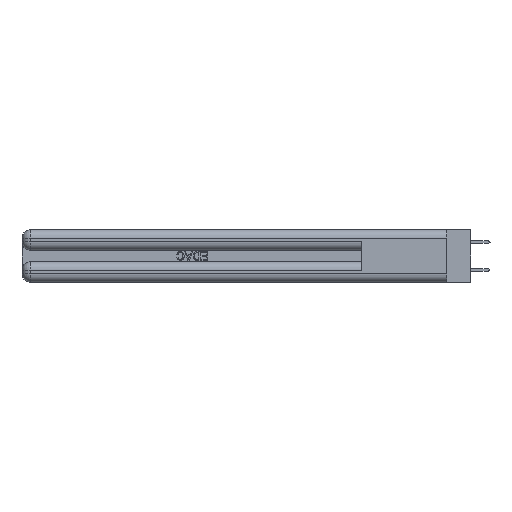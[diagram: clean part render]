
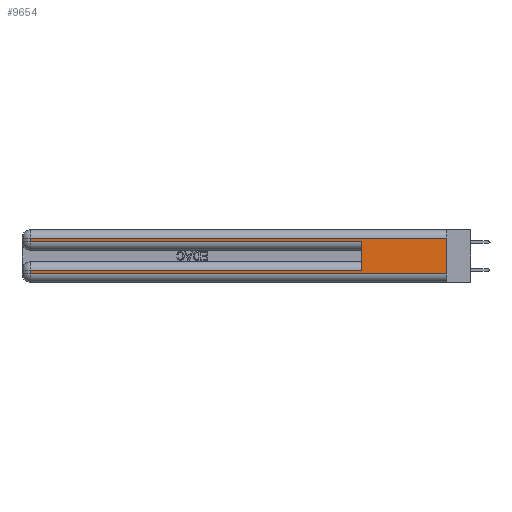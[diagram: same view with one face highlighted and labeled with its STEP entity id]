
A CAD part, left-side view. The second image highlights one B-rep face of the part: STEP entity #9654.
In plain terms, the highlighted planar face has unit normal (-1, 0, 0).
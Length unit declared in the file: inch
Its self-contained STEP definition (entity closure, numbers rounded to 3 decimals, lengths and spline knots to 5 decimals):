
#484 = CARTESIAN_POINT ( 'NONE',  ( 0., 0.6, 0.145 ) ) ;
#1124 = CARTESIAN_POINT ( 'NONE',  ( 0., 2.94, 0.37 ) ) ;
#2005 = VERTEX_POINT ( 'NONE', #11584 ) ;
#2171 = LINE ( 'NONE', #6104, #13094 ) ;
#2216 = DIRECTION ( 'NONE',  ( 0., 0., -1. ) ) ;
#2719 = VECTOR ( 'NONE', #2216, 39.37008 ) ;
#3915 = ORIENTED_EDGE ( 'NONE', *, *, #27995, .T. ) ;
#4435 = EDGE_CURVE ( 'NONE', #2005, #12462, #10075, .T. ) ;
#5364 = DIRECTION ( 'NONE',  ( 1., 0., 0. ) ) ;
#6104 = CARTESIAN_POINT ( 'NONE',  ( 0., 0., 0.06 ) ) ;
#6538 = ORIENTED_EDGE ( 'NONE', *, *, #22815, .T. ) ;
#6700 = EDGE_CURVE ( 'NONE', #31716, #38240, #8829, .T. ) ;
#7305 = DIRECTION ( 'NONE',  ( 0., -1., 0. ) ) ;
#7788 = CARTESIAN_POINT ( 'NONE',  ( 0., 2.94, 0.37 ) ) ;
#8379 = VECTOR ( 'NONE', #30984, 39.37008 ) ;
#8384 = DIRECTION ( 'NONE',  ( 0., -1., 0. ) ) ;
#8829 = LINE ( 'NONE', #21526, #8379 ) ;
#9579 = ORIENTED_EDGE ( 'NONE', *, *, #6700, .T. ) ;
#9654 = ADVANCED_FACE ( 'NONE', ( #11792 ), #26966, .F. ) ;
#9795 = VECTOR ( 'NONE', #15200, 39.37008 ) ;
#9812 = LINE ( 'NONE', #32576, #33834 ) ;
#10075 = LINE ( 'NONE', #484, #14233 ) ;
#11584 = CARTESIAN_POINT ( 'NONE',  ( 0., 0.6, 0.085 ) ) ;
#11792 = FACE_OUTER_BOUND ( 'NONE', #14439, .T. ) ;
#12462 = VERTEX_POINT ( 'NONE', #17905 ) ;
#12486 = EDGE_CURVE ( 'NONE', #35763, #12462, #9812, .T. ) ;
#13094 = VECTOR ( 'NONE', #8384, 39.37008 ) ;
#13148 = AXIS2_PLACEMENT_3D ( 'NONE', #36479, #5364, #20777 ) ;
#14137 = ORIENTED_EDGE ( 'NONE', *, *, #4435, .F. ) ;
#14233 = VECTOR ( 'NONE', #20050, 39.37008 ) ;
#14439 = EDGE_LOOP ( 'NONE', ( #24627, #9579, #3915, #22885, #14137, #6538, #19236, #23419 ) ) ;
#15200 = DIRECTION ( 'NONE',  ( 0., 1., 0. ) ) ;
#15287 = LINE ( 'NONE', #21546, #2719 ) ;
#16349 = VERTEX_POINT ( 'NONE', #16512 ) ;
#16512 = CARTESIAN_POINT ( 'NONE',  ( 0., 2.94, 0.085 ) ) ;
#17905 = CARTESIAN_POINT ( 'NONE',  ( 0., 0.6, 0.285 ) ) ;
#18351 = LINE ( 'NONE', #28795, #9795 ) ;
#19073 = CARTESIAN_POINT ( 'NONE',  ( 0., 2.94, 0.31 ) ) ;
#19236 = ORIENTED_EDGE ( 'NONE', *, *, #37126, .T. ) ;
#19526 = CARTESIAN_POINT ( 'NONE',  ( 0., 2.94, 0.285 ) ) ;
#20050 = DIRECTION ( 'NONE',  ( 0., 0., 1. ) ) ;
#20777 = DIRECTION ( 'NONE',  ( 0., 0., -1. ) ) ;
#21146 = CARTESIAN_POINT ( 'NONE',  ( 0., 2.94, 0.06 ) ) ;
#21526 = CARTESIAN_POINT ( 'NONE',  ( 0., 0., 0.31 ) ) ;
#21546 = CARTESIAN_POINT ( 'NONE',  ( 0., 0., 0.37 ) ) ;
#21895 = VECTOR ( 'NONE', #39509, 39.37008 ) ;
#22815 = EDGE_CURVE ( 'NONE', #2005, #16349, #18351, .T. ) ;
#22885 = ORIENTED_EDGE ( 'NONE', *, *, #12486, .T. ) ;
#23309 = EDGE_CURVE ( 'NONE', #33878, #38286, #2171, .T. ) ;
#23384 = LINE ( 'NONE', #7788, #21895 ) ;
#23419 = ORIENTED_EDGE ( 'NONE', *, *, #23309, .T. ) ;
#24627 = ORIENTED_EDGE ( 'NONE', *, *, #29387, .F. ) ;
#26156 = VECTOR ( 'NONE', #29727, 39.37008 ) ;
#26966 = PLANE ( 'NONE',  #13148 ) ;
#27995 = EDGE_CURVE ( 'NONE', #38240, #35763, #23384, .T. ) ;
#28795 = CARTESIAN_POINT ( 'NONE',  ( 0., 0., 0.085 ) ) ;
#29387 = EDGE_CURVE ( 'NONE', #31716, #38286, #15287, .T. ) ;
#29528 = LINE ( 'NONE', #1124, #26156 ) ;
#29727 = DIRECTION ( 'NONE',  ( 0., 0., -1. ) ) ;
#30984 = DIRECTION ( 'NONE',  ( 0., 1., 0. ) ) ;
#31716 = VERTEX_POINT ( 'NONE', #38873 ) ;
#32576 = CARTESIAN_POINT ( 'NONE',  ( 0., 0., 0.285 ) ) ;
#33834 = VECTOR ( 'NONE', #7305, 39.37008 ) ;
#33878 = VERTEX_POINT ( 'NONE', #21146 ) ;
#35763 = VERTEX_POINT ( 'NONE', #19526 ) ;
#36479 = CARTESIAN_POINT ( 'NONE',  ( 0., 0., 0.37 ) ) ;
#37126 = EDGE_CURVE ( 'NONE', #16349, #33878, #29528, .T. ) ;
#38240 = VERTEX_POINT ( 'NONE', #19073 ) ;
#38286 = VERTEX_POINT ( 'NONE', #38499 ) ;
#38499 = CARTESIAN_POINT ( 'NONE',  ( 0., 0., 0.06 ) ) ;
#38873 = CARTESIAN_POINT ( 'NONE',  ( 0., 0., 0.31 ) ) ;
#39509 = DIRECTION ( 'NONE',  ( 0., 0., -1. ) ) ;
